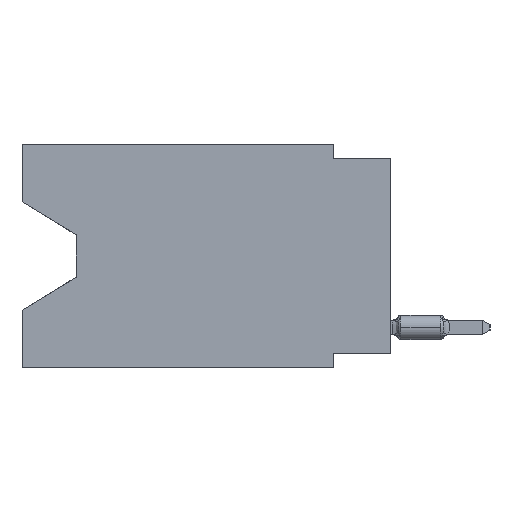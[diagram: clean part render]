
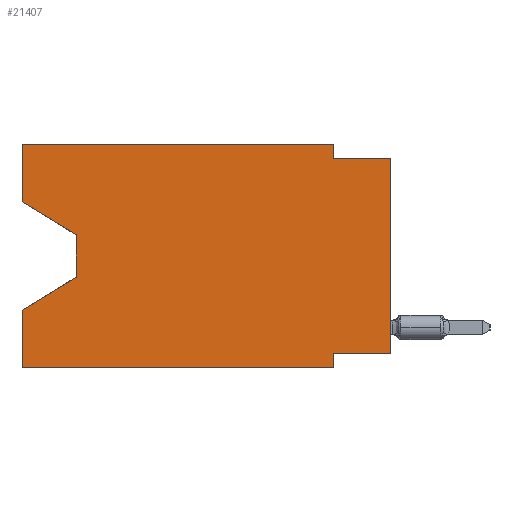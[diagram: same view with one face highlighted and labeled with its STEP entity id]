
A CAD part, left-side view. The second image highlights one B-rep face of the part: STEP entity #21407.
In plain terms, the highlighted planar face has unit normal (-1, 0, 0).
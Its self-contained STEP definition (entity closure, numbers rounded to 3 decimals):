
#75 = VECTOR ( 'NONE', #57502, 1000. ) ;
#957 = CARTESIAN_POINT ( 'NONE',  ( 0., 16.383, 0. ) ) ;
#962 = LINE ( 'NONE', #27848, #63650 ) ;
#1367 = VERTEX_POINT ( 'NONE', #19719 ) ;
#1599 = ORIENTED_EDGE ( 'NONE', *, *, #17981, .F. ) ;
#1826 = EDGE_CURVE ( 'NONE', #33454, #55159, #36343, .T. ) ;
#1981 = VERTEX_POINT ( 'NONE', #68751 ) ;
#2696 = DIRECTION ( 'NONE',  ( 0., -0.855, -0.519 ) ) ;
#3574 = CARTESIAN_POINT ( 'NONE',  ( 0., 0., -9.271 ) ) ;
#3721 = LINE ( 'NONE', #55701, #23396 ) ;
#4041 = ORIENTED_EDGE ( 'NONE', *, *, #59510, .T. ) ;
#5602 = LINE ( 'NONE', #58279, #38340 ) ;
#6730 = CARTESIAN_POINT ( 'NONE',  ( 0., 16.383, -7.36 ) ) ;
#6862 = CARTESIAN_POINT ( 'NONE',  ( 0., 2.54, 0. ) ) ;
#7228 = ORIENTED_EDGE ( 'NONE', *, *, #58728, .F. ) ;
#7686 = VECTOR ( 'NONE', #58848, 1000. ) ;
#7929 = EDGE_CURVE ( 'NONE', #47497, #1981, #5602, .T. ) ;
#8104 = CARTESIAN_POINT ( 'NONE',  ( 0., 16.383, 0. ) ) ;
#9935 = ORIENTED_EDGE ( 'NONE', *, *, #13890, .T. ) ;
#10503 = DIRECTION ( 'NONE',  ( 0., 0., -1. ) ) ;
#13890 = EDGE_CURVE ( 'NONE', #33454, #36243, #68048, .T. ) ;
#14666 = ORIENTED_EDGE ( 'NONE', *, *, #23768, .T. ) ;
#15349 = EDGE_LOOP ( 'NONE', ( #4041, #33455, #14666, #7228, #63809, #39660, #15802, #9935, #58492, #41726, #15689, #1599 ) ) ;
#15689 = ORIENTED_EDGE ( 'NONE', *, *, #58727, .F. ) ;
#15802 = ORIENTED_EDGE ( 'NONE', *, *, #1826, .F. ) ;
#17138 = CARTESIAN_POINT ( 'NONE',  ( 0., 0., -0.635 ) ) ;
#17981 = EDGE_CURVE ( 'NONE', #64398, #27086, #67281, .T. ) ;
#18809 = DIRECTION ( 'NONE',  ( 0., 0., -1. ) ) ;
#19719 = CARTESIAN_POINT ( 'NONE',  ( 0., 13.97, -5.893 ) ) ;
#20313 = CARTESIAN_POINT ( 'NONE',  ( 0., 16.383, 0. ) ) ;
#21407 = ADVANCED_FACE ( 'NONE', ( #31164 ), #25609, .F. ) ;
#21907 = CARTESIAN_POINT ( 'NONE',  ( 0., 13.97, -4.013 ) ) ;
#23385 = EDGE_CURVE ( 'NONE', #55159, #34788, #66923, .T. ) ;
#23396 = VECTOR ( 'NONE', #2696, 1000. ) ;
#23768 = EDGE_CURVE ( 'NONE', #1367, #37483, #55335, .T. ) ;
#24375 = EDGE_CURVE ( 'NONE', #1981, #36243, #48024, .T. ) ;
#25609 = PLANE ( 'NONE',  #25984 ) ;
#25984 = AXIS2_PLACEMENT_3D ( 'NONE', #29802, #46503, #30825 ) ;
#26808 = DIRECTION ( 'NONE',  ( 0., -1., 0. ) ) ;
#27086 = VERTEX_POINT ( 'NONE', #957 ) ;
#27848 = CARTESIAN_POINT ( 'NONE',  ( 0., 16.383, -9.906 ) ) ;
#28786 = VERTEX_POINT ( 'NONE', #68368 ) ;
#29802 = CARTESIAN_POINT ( 'NONE',  ( 0., 16.383, 0. ) ) ;
#30825 = DIRECTION ( 'NONE',  ( 0., 0., -1. ) ) ;
#31164 = FACE_OUTER_BOUND ( 'NONE', #15349, .T. ) ;
#31911 = CARTESIAN_POINT ( 'NONE',  ( 0., 0., -9.271 ) ) ;
#33454 = VERTEX_POINT ( 'NONE', #31911 ) ;
#33455 = ORIENTED_EDGE ( 'NONE', *, *, #61240, .T. ) ;
#34392 = CARTESIAN_POINT ( 'NONE',  ( 0., 13.97, -5.893 ) ) ;
#34788 = VERTEX_POINT ( 'NONE', #40872 ) ;
#35103 = DIRECTION ( 'NONE',  ( 0., 0.855, -0.519 ) ) ;
#35863 = CARTESIAN_POINT ( 'NONE',  ( 0., 2.54, -9.271 ) ) ;
#36243 = VERTEX_POINT ( 'NONE', #17138 ) ;
#36319 = DIRECTION ( 'NONE',  ( 0., 0., 1. ) ) ;
#36343 = LINE ( 'NONE', #3574, #55585 ) ;
#37483 = VERTEX_POINT ( 'NONE', #6730 ) ;
#37556 = CARTESIAN_POINT ( 'NONE',  ( 0., 0., -0.635 ) ) ;
#37630 = VECTOR ( 'NONE', #56573, 1000. ) ;
#38340 = VECTOR ( 'NONE', #10503, 1000. ) ;
#38805 = VECTOR ( 'NONE', #35103, 1000. ) ;
#38821 = VECTOR ( 'NONE', #36319, 1000. ) ;
#39660 = ORIENTED_EDGE ( 'NONE', *, *, #23385, .F. ) ;
#40863 = LINE ( 'NONE', #20313, #40972 ) ;
#40872 = CARTESIAN_POINT ( 'NONE',  ( 0., 2.54, -9.906 ) ) ;
#40972 = VECTOR ( 'NONE', #67044, 1000. ) ;
#41216 = DIRECTION ( 'NONE',  ( 0., 1., 0. ) ) ;
#41726 = ORIENTED_EDGE ( 'NONE', *, *, #7929, .F. ) ;
#46029 = VECTOR ( 'NONE', #62924, 1000. ) ;
#46503 = DIRECTION ( 'NONE',  ( 1., 0., 0. ) ) ;
#47497 = VERTEX_POINT ( 'NONE', #6862 ) ;
#48024 = LINE ( 'NONE', #37556, #7686 ) ;
#48621 = VERTEX_POINT ( 'NONE', #21907 ) ;
#50193 = CARTESIAN_POINT ( 'NONE',  ( 0., 2.54, -9.906 ) ) ;
#51001 = VECTOR ( 'NONE', #18809, 1000. ) ;
#55159 = VERTEX_POINT ( 'NONE', #35863 ) ;
#55335 = LINE ( 'NONE', #34392, #38805 ) ;
#55585 = VECTOR ( 'NONE', #41216, 1000. ) ;
#55701 = CARTESIAN_POINT ( 'NONE',  ( 0., 16.383, -2.546 ) ) ;
#56573 = DIRECTION ( 'NONE',  ( 0., 0., 1. ) ) ;
#57502 = DIRECTION ( 'NONE',  ( 0., 0., 1. ) ) ;
#57828 = CARTESIAN_POINT ( 'NONE',  ( 0., 16.383, 0. ) ) ;
#58040 = CARTESIAN_POINT ( 'NONE',  ( 0., 13.97, -4.013 ) ) ;
#58279 = CARTESIAN_POINT ( 'NONE',  ( 0., 2.54, 0. ) ) ;
#58386 = LINE ( 'NONE', #58040, #46029 ) ;
#58492 = ORIENTED_EDGE ( 'NONE', *, *, #24375, .F. ) ;
#58727 = EDGE_CURVE ( 'NONE', #27086, #47497, #40863, .T. ) ;
#58728 = EDGE_CURVE ( 'NONE', #28786, #37483, #62134, .T. ) ;
#58848 = DIRECTION ( 'NONE',  ( 0., -1., 0. ) ) ;
#59510 = EDGE_CURVE ( 'NONE', #64398, #48621, #3721, .T. ) ;
#61240 = EDGE_CURVE ( 'NONE', #48621, #1367, #58386, .T. ) ;
#62134 = LINE ( 'NONE', #8104, #37630 ) ;
#62924 = DIRECTION ( 'NONE',  ( 0., 0., -1. ) ) ;
#63499 = CARTESIAN_POINT ( 'NONE',  ( 0., 0., 0. ) ) ;
#63650 = VECTOR ( 'NONE', #26808, 1000. ) ;
#63809 = ORIENTED_EDGE ( 'NONE', *, *, #67532, .T. ) ;
#64398 = VERTEX_POINT ( 'NONE', #67286 ) ;
#66923 = LINE ( 'NONE', #50193, #51001 ) ;
#67044 = DIRECTION ( 'NONE',  ( 0., -1., 0. ) ) ;
#67281 = LINE ( 'NONE', #57828, #75 ) ;
#67286 = CARTESIAN_POINT ( 'NONE',  ( 0., 16.383, -2.546 ) ) ;
#67532 = EDGE_CURVE ( 'NONE', #28786, #34788, #962, .T. ) ;
#68048 = LINE ( 'NONE', #63499, #38821 ) ;
#68368 = CARTESIAN_POINT ( 'NONE',  ( 0., 16.383, -9.906 ) ) ;
#68751 = CARTESIAN_POINT ( 'NONE',  ( 0., 2.54, -0.635 ) ) ;
